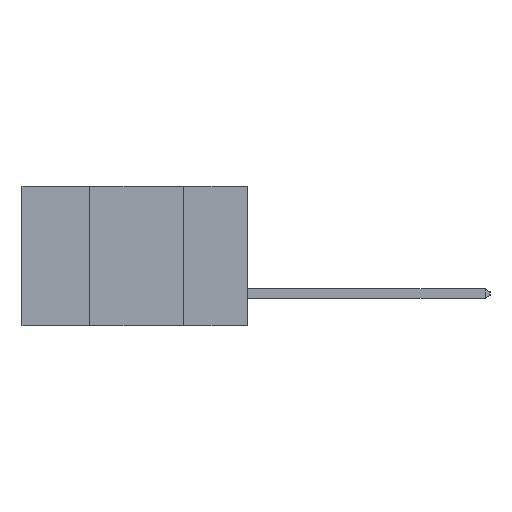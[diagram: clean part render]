
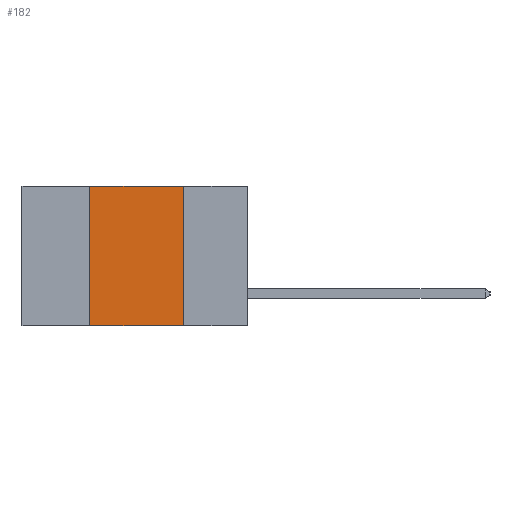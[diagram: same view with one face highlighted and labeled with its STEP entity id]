
A CAD part, left-side view. The second image highlights one B-rep face of the part: STEP entity #182.
In plain terms, the highlighted planar face has unit normal (-1, 0, 0).
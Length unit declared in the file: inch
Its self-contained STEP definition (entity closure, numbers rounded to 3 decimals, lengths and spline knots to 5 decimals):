
#182 = ADVANCED_FACE ( 'NONE', ( #4515 ), #15176, .F. ) ;
#303 = VECTOR ( 'NONE', #2615, 39.37008 ) ;
#319 = LINE ( 'NONE', #8725, #16416 ) ;
#1166 = CARTESIAN_POINT ( 'NONE',  ( 0., 0.6, 0. ) ) ;
#1329 = EDGE_LOOP ( 'NONE', ( #11744, #14087, #18608, #16983 ) ) ;
#2615 = DIRECTION ( 'NONE',  ( 0., -1., 0. ) ) ;
#2813 = CARTESIAN_POINT ( 'NONE',  ( 0., 0.6, -0.37 ) ) ;
#3975 = EDGE_CURVE ( 'NONE', #15501, #6872, #5125, .T. ) ;
#4515 = FACE_OUTER_BOUND ( 'NONE', #1329, .T. ) ;
#5125 = LINE ( 'NONE', #18940, #9287 ) ;
#6418 = DIRECTION ( 'NONE',  ( 0., 0., -1. ) ) ;
#6872 = VERTEX_POINT ( 'NONE', #8550 ) ;
#7156 = EDGE_CURVE ( 'NONE', #15501, #16949, #12771, .T. ) ;
#7372 = DIRECTION ( 'NONE',  ( 0., -1., 0. ) ) ;
#7702 = CARTESIAN_POINT ( 'NONE',  ( 0., 0.17, -0.37 ) ) ;
#8550 = CARTESIAN_POINT ( 'NONE',  ( 0., 0.42, 0. ) ) ;
#8725 = CARTESIAN_POINT ( 'NONE',  ( 0., 0.17, -0.37 ) ) ;
#9287 = VECTOR ( 'NONE', #19099, 39.37008 ) ;
#10262 = DIRECTION ( 'NONE',  ( 1., 0., 0. ) ) ;
#10397 = VECTOR ( 'NONE', #7372, 39.37008 ) ;
#10875 = LINE ( 'NONE', #1166, #10397 ) ;
#10956 = CARTESIAN_POINT ( 'NONE',  ( 0., 0.42, -0.37 ) ) ;
#11168 = CARTESIAN_POINT ( 'NONE',  ( 0., 0.17, 0. ) ) ;
#11744 = ORIENTED_EDGE ( 'NONE', *, *, #12113, .F. ) ;
#12113 = EDGE_CURVE ( 'NONE', #19539, #16949, #319, .T. ) ;
#12771 = LINE ( 'NONE', #2813, #303 ) ;
#14087 = ORIENTED_EDGE ( 'NONE', *, *, #16295, .F. ) ;
#15076 = DIRECTION ( 'NONE',  ( 0., 0., -1. ) ) ;
#15130 = CARTESIAN_POINT ( 'NONE',  ( 0., 0.6, 0. ) ) ;
#15176 = PLANE ( 'NONE',  #17074 ) ;
#15501 = VERTEX_POINT ( 'NONE', #10956 ) ;
#16295 = EDGE_CURVE ( 'NONE', #6872, #19539, #10875, .T. ) ;
#16416 = VECTOR ( 'NONE', #6418, 39.37008 ) ;
#16949 = VERTEX_POINT ( 'NONE', #7702 ) ;
#16983 = ORIENTED_EDGE ( 'NONE', *, *, #7156, .T. ) ;
#17074 = AXIS2_PLACEMENT_3D ( 'NONE', #15130, #10262, #15076 ) ;
#18608 = ORIENTED_EDGE ( 'NONE', *, *, #3975, .F. ) ;
#18940 = CARTESIAN_POINT ( 'NONE',  ( 0., 0.42, -0.37 ) ) ;
#19099 = DIRECTION ( 'NONE',  ( 0., 0., 1. ) ) ;
#19539 = VERTEX_POINT ( 'NONE', #11168 ) ;
